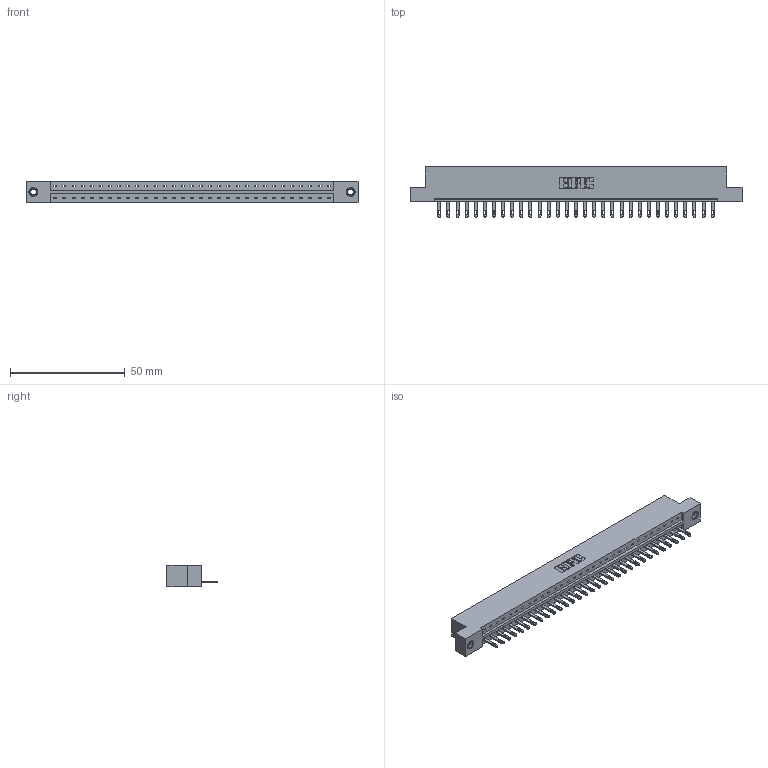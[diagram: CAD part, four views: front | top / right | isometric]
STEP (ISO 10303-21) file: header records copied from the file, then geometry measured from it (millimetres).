
FILE_DESCRIPTION (( 'STEP AP203' ), '1' );
FILE_NAME ('333-031-500-107.STEP', '2018-08-02T19:05:52', ( '' ), ( '' ), 'SwSTEP 2.0', 'SolidWorks 2016', '' );
FILE_SCHEMA (( 'CONFIG_CONTROL_DESIGN' ));
Length unit declared in the file: inch
Products named in the file (4): 333 Part_Flush - .156 Dia - TI; 345-292-001_345-293-100; 345-250-001_345-250-005-103; 333-031-500-107
Assembly tree (34 placements, depth 2):
  333-031-500-107
    333 Part_Flush - .156 Dia - TI
    345-292-001_345-293-100  x31
    345-250-001_345-250-005-103  x2
Bounding box: 144.37 x 21.85 x 9.4 mm (x, y, z)
Volume: 14439.1 mm3; surface area: 15663.7 mm2
Topology: 34 solids, 34 shells, 1848 faces, 5655 edges, 3762 vertices
Faces by surface type: plane 1218, cylinder 614, cone 12, torus 4
Entity records: 21490 total; most frequent: CARTESIAN_POINT 3690, ORIENTED_EDGE 3650, DIRECTION 3169, EDGE_CURVE 1825, VECTOR 1673, LINE 1673, VERTEX_POINT 1212, AXIS2_PLACEMENT_3D 748
